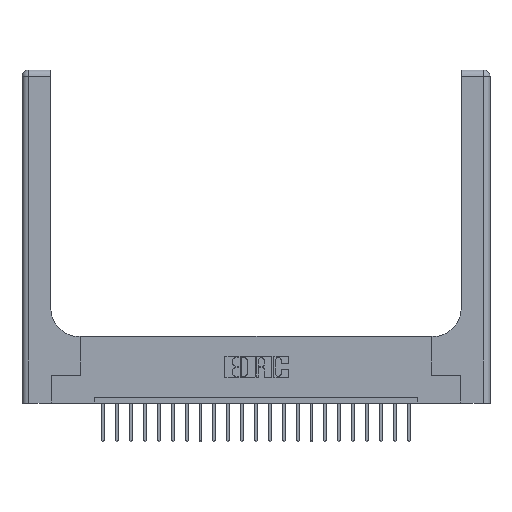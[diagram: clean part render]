
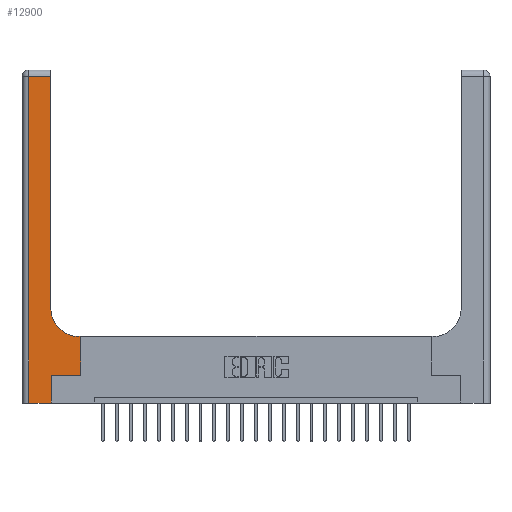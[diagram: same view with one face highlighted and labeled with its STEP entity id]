
A CAD part, top view. The second image highlights one B-rep face of the part: STEP entity #12900.
In plain terms, the highlighted planar face has unit normal (0, 0, 1).
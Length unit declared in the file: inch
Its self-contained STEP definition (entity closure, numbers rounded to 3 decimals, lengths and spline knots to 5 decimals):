
#649 = LINE ( 'NONE', #12832, #9778 ) ;
#942 = LINE ( 'NONE', #10847, #20357 ) ;
#973 = CARTESIAN_POINT ( 'NONE',  ( 0.528, 0.25, 0.37 ) ) ;
#1108 = CARTESIAN_POINT ( 'NONE',  ( 0.26, 0.6, 0.37 ) ) ;
#1537 = DIRECTION ( 'NONE',  ( 1., 0., 0. ) ) ;
#1547 = FACE_OUTER_BOUND ( 'NONE', #20886, .T. ) ;
#2646 = ORIENTED_EDGE ( 'NONE', *, *, #11610, .T. ) ;
#3402 = VERTEX_POINT ( 'NONE', #973 ) ;
#3411 = VERTEX_POINT ( 'NONE', #7920 ) ;
#4142 = VECTOR ( 'NONE', #21930, 39.37008 ) ;
#4254 = VECTOR ( 'NONE', #18967, 39.37008 ) ;
#4884 = CARTESIAN_POINT ( 'NONE',  ( 0., 2.94, 0.37 ) ) ;
#5160 = ORIENTED_EDGE ( 'NONE', *, *, #17182, .T. ) ;
#5267 = CARTESIAN_POINT ( 'NONE',  ( 0.51, 0.6, 0.37 ) ) ;
#5935 = ORIENTED_EDGE ( 'NONE', *, *, #14370, .T. ) ;
#6047 = DIRECTION ( 'NONE',  ( 1., 0., 0. ) ) ;
#6235 = AXIS2_PLACEMENT_3D ( 'NONE', #9340, #14578, #6047 ) ;
#6334 = ORIENTED_EDGE ( 'NONE', *, *, #18866, .T. ) ;
#6609 = CIRCLE ( 'NONE', #6235, 0.25 ) ;
#7379 = DIRECTION ( 'NONE',  ( 0., 1., 0. ) ) ;
#7506 = CARTESIAN_POINT ( 'NONE',  ( 0.06, 2.94, 0.37 ) ) ;
#7920 = CARTESIAN_POINT ( 'NONE',  ( 0.265, 0., 0.37 ) ) ;
#7987 = CARTESIAN_POINT ( 'NONE',  ( 0.528, 0.6, 0.37 ) ) ;
#7995 = VECTOR ( 'NONE', #17506, 39.37008 ) ;
#8185 = CARTESIAN_POINT ( 'NONE',  ( 0.265, 0.25, 0.37 ) ) ;
#8324 = VERTEX_POINT ( 'NONE', #7987 ) ;
#8405 = CARTESIAN_POINT ( 'NONE',  ( 0.26, 0.85, 0.37 ) ) ;
#8570 = VECTOR ( 'NONE', #14981, 39.37008 ) ;
#8996 = LINE ( 'NONE', #10699, #18041 ) ;
#9079 = VECTOR ( 'NONE', #1537, 39.37008 ) ;
#9340 = CARTESIAN_POINT ( 'NONE',  ( 0.51, 0.85, 0.37 ) ) ;
#9652 = LINE ( 'NONE', #13075, #4142 ) ;
#9778 = VECTOR ( 'NONE', #7379, 39.37008 ) ;
#9847 = ORIENTED_EDGE ( 'NONE', *, *, #22045, .T. ) ;
#9860 = VERTEX_POINT ( 'NONE', #16878 ) ;
#10499 = EDGE_CURVE ( 'NONE', #8324, #17595, #18282, .T. ) ;
#10562 = CARTESIAN_POINT ( 'NONE',  ( 0.26, 3., 0.37 ) ) ;
#10699 = CARTESIAN_POINT ( 'NONE',  ( 0.265, 0., 0.37 ) ) ;
#10847 = CARTESIAN_POINT ( 'NONE',  ( 0.265, 0.25, 0.37 ) ) ;
#11610 = EDGE_CURVE ( 'NONE', #3411, #15269, #8996, .T. ) ;
#11881 = LINE ( 'NONE', #18820, #9079 ) ;
#12399 = CARTESIAN_POINT ( 'NONE',  ( 0.26, 2.94, 0.37 ) ) ;
#12832 = CARTESIAN_POINT ( 'NONE',  ( 0.528, 0.25, 0.37 ) ) ;
#12900 = ADVANCED_FACE ( 'NONE', ( #1547 ), #13712, .F. ) ;
#13075 = CARTESIAN_POINT ( 'NONE',  ( 0.06, 3., 0.37 ) ) ;
#13173 = ORIENTED_EDGE ( 'NONE', *, *, #21896, .T. ) ;
#13712 = PLANE ( 'NONE',  #20261 ) ;
#14207 = VERTEX_POINT ( 'NONE', #8405 ) ;
#14334 = DIRECTION ( 'NONE',  ( 0., 1., 0. ) ) ;
#14370 = EDGE_CURVE ( 'NONE', #3402, #8324, #649, .T. ) ;
#14444 = ORIENTED_EDGE ( 'NONE', *, *, #10499, .T. ) ;
#14480 = DIRECTION ( 'NONE',  ( 1., 0., 0. ) ) ;
#14578 = DIRECTION ( 'NONE',  ( 0., 0., -1. ) ) ;
#14972 = CARTESIAN_POINT ( 'NONE',  ( 0., 3., 0.37 ) ) ;
#14981 = DIRECTION ( 'NONE',  ( -1., 0., 0. ) ) ;
#15225 = LINE ( 'NONE', #4884, #4254 ) ;
#15269 = VERTEX_POINT ( 'NONE', #8185 ) ;
#15461 = EDGE_CURVE ( 'NONE', #14207, #20544, #19193, .T. ) ;
#16878 = CARTESIAN_POINT ( 'NONE',  ( 0.06, 0., 0.37 ) ) ;
#17182 = EDGE_CURVE ( 'NONE', #9860, #3411, #11881, .T. ) ;
#17388 = EDGE_CURVE ( 'NONE', #15269, #3402, #942, .T. ) ;
#17506 = DIRECTION ( 'NONE',  ( 0., 1., 0. ) ) ;
#17595 = VERTEX_POINT ( 'NONE', #5267 ) ;
#18041 = VECTOR ( 'NONE', #14334, 39.37008 ) ;
#18282 = LINE ( 'NONE', #1108, #8570 ) ;
#18820 = CARTESIAN_POINT ( 'NONE',  ( 0., 0., 0.37 ) ) ;
#18842 = ORIENTED_EDGE ( 'NONE', *, *, #15461, .T. ) ;
#18866 = EDGE_CURVE ( 'NONE', #17595, #14207, #6609, .T. ) ;
#18967 = DIRECTION ( 'NONE',  ( -1., 0., 0. ) ) ;
#19193 = LINE ( 'NONE', #10562, #7995 ) ;
#19202 = VERTEX_POINT ( 'NONE', #7506 ) ;
#20261 = AXIS2_PLACEMENT_3D ( 'NONE', #14972, #22337, #21899 ) ;
#20357 = VECTOR ( 'NONE', #14480, 39.37008 ) ;
#20544 = VERTEX_POINT ( 'NONE', #12399 ) ;
#20886 = EDGE_LOOP ( 'NONE', ( #18842, #9847, #13173, #5160, #2646, #22186, #5935, #14444, #6334 ) ) ;
#21896 = EDGE_CURVE ( 'NONE', #19202, #9860, #9652, .T. ) ;
#21899 = DIRECTION ( 'NONE',  ( -1., 0., 0. ) ) ;
#21930 = DIRECTION ( 'NONE',  ( 0., -1., 0. ) ) ;
#22045 = EDGE_CURVE ( 'NONE', #20544, #19202, #15225, .T. ) ;
#22186 = ORIENTED_EDGE ( 'NONE', *, *, #17388, .T. ) ;
#22337 = DIRECTION ( 'NONE',  ( 0., 0., -1. ) ) ;
